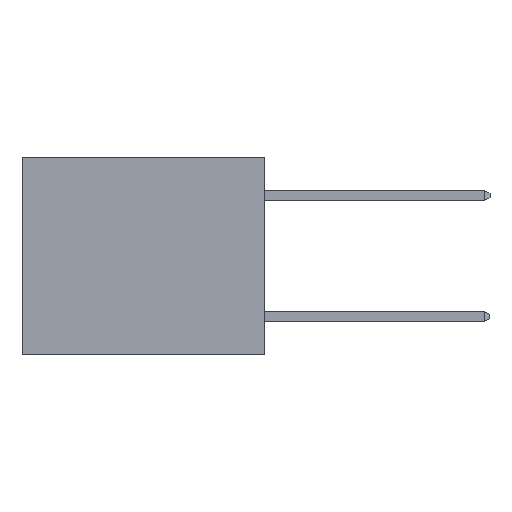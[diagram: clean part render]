
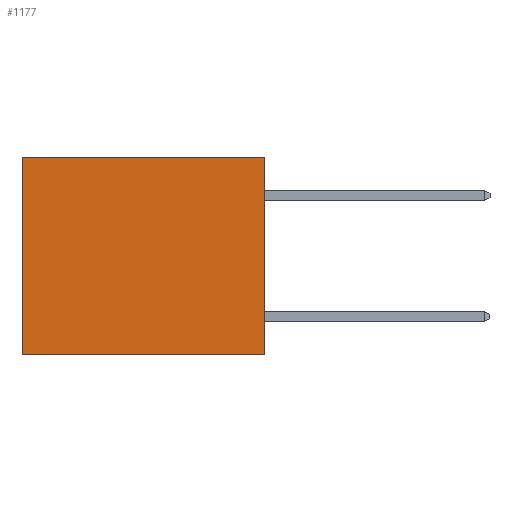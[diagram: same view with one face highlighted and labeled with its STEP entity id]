
A CAD part, left-side view. The second image highlights one B-rep face of the part: STEP entity #1177.
In plain terms, the highlighted planar face has unit normal (-1, 0, 0).
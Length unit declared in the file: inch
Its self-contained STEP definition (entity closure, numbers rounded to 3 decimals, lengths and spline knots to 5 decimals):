
#217 = VECTOR ( 'NONE', #10897, 39.37008 ) ;
#379 = DIRECTION ( 'NONE',  ( 1., 0., 0. ) ) ;
#511 = CARTESIAN_POINT ( 'NONE',  ( 0.3165, 0., -0.49 ) ) ;
#577 = CARTESIAN_POINT ( 'NONE',  ( 0.3165, 0.6, -0.49 ) ) ;
#909 = ORIENTED_EDGE ( 'NONE', *, *, #5020, .F. ) ;
#1177 = ADVANCED_FACE ( 'NONE', ( #11613 ), #5202, .F. ) ;
#1403 = EDGE_CURVE ( 'NONE', #4440, #12491, #13832, .T. ) ;
#1753 = DIRECTION ( 'NONE',  ( 0., 1., 0. ) ) ;
#2892 = VECTOR ( 'NONE', #13572, 39.37008 ) ;
#3129 = EDGE_CURVE ( 'NONE', #15413, #4411, #12114, .T. ) ;
#4056 = CARTESIAN_POINT ( 'NONE',  ( 0.3165, 0., -0.49 ) ) ;
#4411 = VERTEX_POINT ( 'NONE', #6061 ) ;
#4417 = EDGE_CURVE ( 'NONE', #4411, #12491, #6088, .T. ) ;
#4440 = VERTEX_POINT ( 'NONE', #12270 ) ;
#4766 = DIRECTION ( 'NONE',  ( 0., 0., -1. ) ) ;
#4917 = CARTESIAN_POINT ( 'NONE',  ( 0.3165, 0.6, -0.49 ) ) ;
#5020 = EDGE_CURVE ( 'NONE', #15413, #4440, #10939, .T. ) ;
#5202 = PLANE ( 'NONE',  #7085 ) ;
#5469 = CARTESIAN_POINT ( 'NONE',  ( 0.3165, 0., 0. ) ) ;
#6061 = CARTESIAN_POINT ( 'NONE',  ( 0.3165, 0.6, 0. ) ) ;
#6083 = CARTESIAN_POINT ( 'NONE',  ( 0.3165, 0., -0.49 ) ) ;
#6088 = LINE ( 'NONE', #4917, #2892 ) ;
#6467 = CARTESIAN_POINT ( 'NONE',  ( 0.3165, 0., 0. ) ) ;
#6640 = ORIENTED_EDGE ( 'NONE', *, *, #1403, .F. ) ;
#7085 = AXIS2_PLACEMENT_3D ( 'NONE', #4056, #379, #8753 ) ;
#7391 = VECTOR ( 'NONE', #4766, 39.37008 ) ;
#7804 = VECTOR ( 'NONE', #1753, 39.37008 ) ;
#8025 = ORIENTED_EDGE ( 'NONE', *, *, #3129, .T. ) ;
#8753 = DIRECTION ( 'NONE',  ( 0., 0., -1. ) ) ;
#10897 = DIRECTION ( 'NONE',  ( 0., 1., 0. ) ) ;
#10939 = LINE ( 'NONE', #511, #7391 ) ;
#11613 = FACE_OUTER_BOUND ( 'NONE', #11998, .T. ) ;
#11998 = EDGE_LOOP ( 'NONE', ( #15140, #6640, #909, #8025 ) ) ;
#12114 = LINE ( 'NONE', #5469, #7804 ) ;
#12270 = CARTESIAN_POINT ( 'NONE',  ( 0.3165, 0., -0.49 ) ) ;
#12491 = VERTEX_POINT ( 'NONE', #577 ) ;
#13572 = DIRECTION ( 'NONE',  ( 0., 0., -1. ) ) ;
#13832 = LINE ( 'NONE', #6083, #217 ) ;
#15140 = ORIENTED_EDGE ( 'NONE', *, *, #4417, .T. ) ;
#15413 = VERTEX_POINT ( 'NONE', #6467 ) ;
